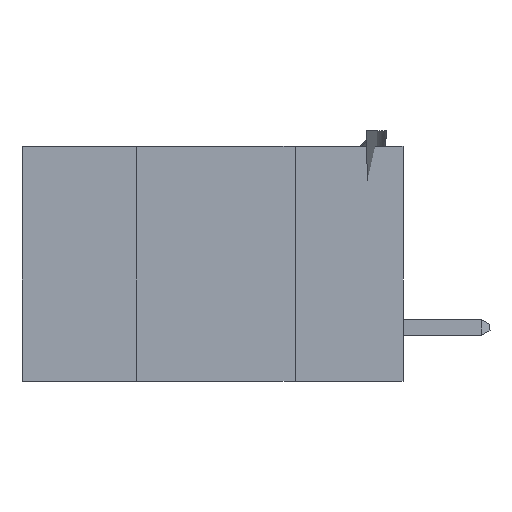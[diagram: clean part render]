
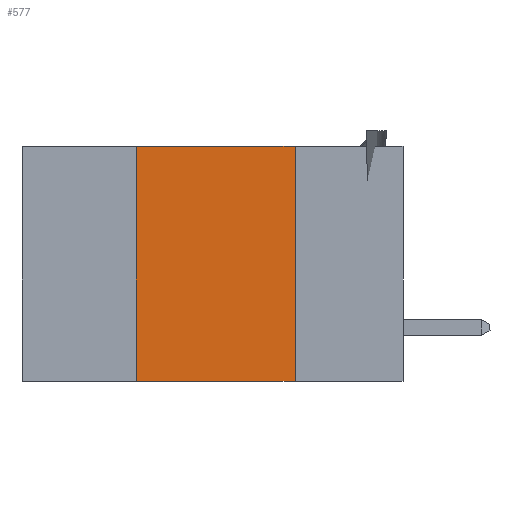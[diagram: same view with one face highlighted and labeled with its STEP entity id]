
A CAD part, left-side view. The second image highlights one B-rep face of the part: STEP entity #577.
In plain terms, the highlighted planar face has unit normal (-1, 0, 0).
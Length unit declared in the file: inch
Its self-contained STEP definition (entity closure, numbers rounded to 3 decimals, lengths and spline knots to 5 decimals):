
#76 = CARTESIAN_POINT ( 'NONE',  ( 0., 0.6, 0. ) ) ;
#93 = VERTEX_POINT ( 'NONE', #3045 ) ;
#250 = ORIENTED_EDGE ( 'NONE', *, *, #6666, .F. ) ;
#549 = DIRECTION ( 'NONE',  ( 1., 0., 0. ) ) ;
#577 = ADVANCED_FACE ( 'NONE', ( #7657 ), #9822, .F. ) ;
#956 = CARTESIAN_POINT ( 'NONE',  ( 0., 0.42, -0.37 ) ) ;
#1070 = CARTESIAN_POINT ( 'NONE',  ( 0., 0.17, 0. ) ) ;
#1172 = DIRECTION ( 'NONE',  ( 0., -1., 0. ) ) ;
#1176 = ORIENTED_EDGE ( 'NONE', *, *, #3462, .T. ) ;
#1300 = CARTESIAN_POINT ( 'NONE',  ( 0., 0.6, -0.37 ) ) ;
#2312 = VECTOR ( 'NONE', #5844, 39.37008 ) ;
#2925 = LINE ( 'NONE', #9344, #9239 ) ;
#2988 = VERTEX_POINT ( 'NONE', #10464 ) ;
#3045 = CARTESIAN_POINT ( 'NONE',  ( 0., 0.42, 0. ) ) ;
#3462 = EDGE_CURVE ( 'NONE', #7398, #2988, #10677, .T. ) ;
#3679 = VECTOR ( 'NONE', #1172, 39.37008 ) ;
#4438 = EDGE_LOOP ( 'NONE', ( #10509, #5771, #250, #1176 ) ) ;
#4448 = VERTEX_POINT ( 'NONE', #1070 ) ;
#5771 = ORIENTED_EDGE ( 'NONE', *, *, #10016, .F. ) ;
#5844 = DIRECTION ( 'NONE',  ( 0., 0., -1. ) ) ;
#6610 = DIRECTION ( 'NONE',  ( 0., 0., 1. ) ) ;
#6666 = EDGE_CURVE ( 'NONE', #7398, #93, #2925, .T. ) ;
#6998 = LINE ( 'NONE', #8888, #2312 ) ;
#7398 = VERTEX_POINT ( 'NONE', #956 ) ;
#7657 = FACE_OUTER_BOUND ( 'NONE', #4438, .T. ) ;
#8078 = DIRECTION ( 'NONE',  ( 0., -1., 0. ) ) ;
#8400 = DIRECTION ( 'NONE',  ( 0., 0., -1. ) ) ;
#8515 = VECTOR ( 'NONE', #8078, 39.37008 ) ;
#8871 = CARTESIAN_POINT ( 'NONE',  ( 0., 0.6, 0. ) ) ;
#8888 = CARTESIAN_POINT ( 'NONE',  ( 0., 0.17, 0. ) ) ;
#9233 = EDGE_CURVE ( 'NONE', #4448, #2988, #6998, .T. ) ;
#9239 = VECTOR ( 'NONE', #6610, 39.37008 ) ;
#9344 = CARTESIAN_POINT ( 'NONE',  ( 0., 0.42, 0. ) ) ;
#9822 = PLANE ( 'NONE',  #10538 ) ;
#9859 = LINE ( 'NONE', #76, #3679 ) ;
#10016 = EDGE_CURVE ( 'NONE', #93, #4448, #9859, .T. ) ;
#10464 = CARTESIAN_POINT ( 'NONE',  ( 0., 0.17, -0.37 ) ) ;
#10509 = ORIENTED_EDGE ( 'NONE', *, *, #9233, .F. ) ;
#10538 = AXIS2_PLACEMENT_3D ( 'NONE', #8871, #549, #8400 ) ;
#10677 = LINE ( 'NONE', #1300, #8515 ) ;
